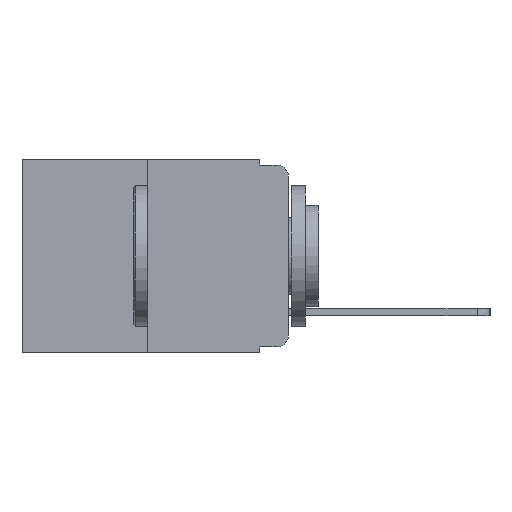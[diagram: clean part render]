
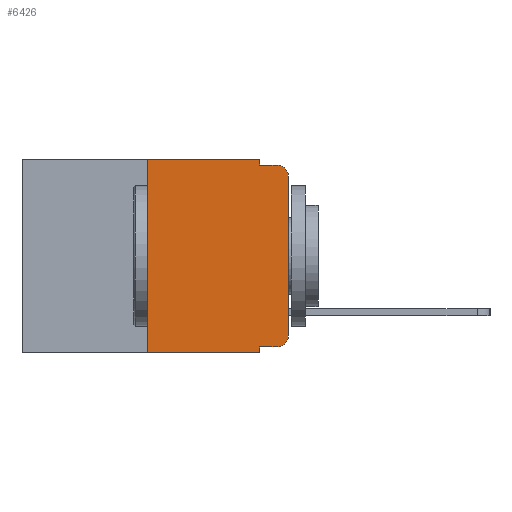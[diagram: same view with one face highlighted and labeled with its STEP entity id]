
A CAD part, left-side view. The second image highlights one B-rep face of the part: STEP entity #6426.
In plain terms, the highlighted planar face has unit normal (-1, 0, 0).
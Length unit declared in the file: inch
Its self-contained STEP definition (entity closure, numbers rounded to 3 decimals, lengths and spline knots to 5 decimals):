
#98 = EDGE_LOOP ( 'NONE', ( #11228, #19823, #4964, #5455, #9560, #14132, #4216, #12463, #16988, #5717 ) ) ;
#233 = CARTESIAN_POINT ( 'NONE',  ( 0., 0.02, -0.01 ) ) ;
#795 = VERTEX_POINT ( 'NONE', #17831 ) ;
#928 = EDGE_CURVE ( 'NONE', #9464, #13873, #5778, .T. ) ;
#1078 = DIRECTION ( 'NONE',  ( 1., 0., 0. ) ) ;
#1104 = VECTOR ( 'NONE', #4983, 39.37008 ) ;
#1154 = VECTOR ( 'NONE', #8101, 39.37008 ) ;
#1570 = LINE ( 'NONE', #16933, #2056 ) ;
#1580 = LINE ( 'NONE', #3253, #1104 ) ;
#1630 = LINE ( 'NONE', #18786, #1154 ) ;
#1838 = DIRECTION ( 'NONE',  ( 0., -1., 0. ) ) ;
#1951 = EDGE_CURVE ( 'NONE', #13873, #5137, #1580, .T. ) ;
#2056 = VECTOR ( 'NONE', #16936, 39.37008 ) ;
#2544 = PLANE ( 'NONE',  #11538 ) ;
#2596 = VECTOR ( 'NONE', #17527, 39.37008 ) ;
#2626 = DIRECTION ( 'NONE',  ( -1., 0., 0. ) ) ;
#2846 = LINE ( 'NONE', #19289, #18240 ) ;
#2942 = DIRECTION ( 'NONE',  ( 0., -1., 0. ) ) ;
#2963 = EDGE_CURVE ( 'NONE', #15920, #5137, #13215, .T. ) ;
#3253 = CARTESIAN_POINT ( 'NONE',  ( 0., 0.051, -0.01 ) ) ;
#3705 = AXIS2_PLACEMENT_3D ( 'NONE', #11559, #11863, #11842 ) ;
#3991 = EDGE_CURVE ( 'NONE', #795, #15920, #1570, .T. ) ;
#4153 = CARTESIAN_POINT ( 'NONE',  ( 0., 0., -0.03 ) ) ;
#4216 = ORIENTED_EDGE ( 'NONE', *, *, #15617, .T. ) ;
#4964 = ORIENTED_EDGE ( 'NONE', *, *, #1951, .F. ) ;
#4983 = DIRECTION ( 'NONE',  ( 0., -1., 0. ) ) ;
#5137 = VERTEX_POINT ( 'NONE', #233 ) ;
#5455 = ORIENTED_EDGE ( 'NONE', *, *, #928, .F. ) ;
#5717 = ORIENTED_EDGE ( 'NONE', *, *, #8567, .T. ) ;
#5778 = LINE ( 'NONE', #17549, #2596 ) ;
#6110 = CARTESIAN_POINT ( 'NONE',  ( 0., 0.473, 0. ) ) ;
#6426 = ADVANCED_FACE ( 'NONE', ( #11651 ), #2544, .F. ) ;
#7258 = VECTOR ( 'NONE', #1838, 39.37008 ) ;
#7268 = CARTESIAN_POINT ( 'NONE',  ( 0., 0.473, 0. ) ) ;
#7919 = VECTOR ( 'NONE', #17334, 39.37008 ) ;
#8100 = CARTESIAN_POINT ( 'NONE',  ( 0., 0.02, -0.333 ) ) ;
#8101 = DIRECTION ( 'NONE',  ( 0., 0., -1. ) ) ;
#8182 = CARTESIAN_POINT ( 'NONE',  ( 0., 0.051, -0.333 ) ) ;
#8341 = CIRCLE ( 'NONE', #19098, 0.02 ) ;
#8567 = EDGE_CURVE ( 'NONE', #12305, #795, #8341, .T. ) ;
#9285 = CARTESIAN_POINT ( 'NONE',  ( 0., 0.25, -0.343 ) ) ;
#9464 = VERTEX_POINT ( 'NONE', #15642 ) ;
#9560 = ORIENTED_EDGE ( 'NONE', *, *, #17837, .F. ) ;
#11228 = ORIENTED_EDGE ( 'NONE', *, *, #3991, .T. ) ;
#11538 = AXIS2_PLACEMENT_3D ( 'NONE', #7268, #1078, #11873 ) ;
#11559 = CARTESIAN_POINT ( 'NONE',  ( 0., 0.02, -0.03 ) ) ;
#11651 = FACE_OUTER_BOUND ( 'NONE', #98, .T. ) ;
#11842 = DIRECTION ( 'NONE',  ( 0., 0., -1. ) ) ;
#11863 = DIRECTION ( 'NONE',  ( -1., 0., 0. ) ) ;
#11873 = DIRECTION ( 'NONE',  ( 0., 0., -1. ) ) ;
#11885 = CARTESIAN_POINT ( 'NONE',  ( 0., 0.02, -0.313 ) ) ;
#11994 = LINE ( 'NONE', #8182, #7919 ) ;
#12085 = LINE ( 'NONE', #6110, #19699 ) ;
#12163 = VERTEX_POINT ( 'NONE', #9285 ) ;
#12305 = VERTEX_POINT ( 'NONE', #8100 ) ;
#12463 = ORIENTED_EDGE ( 'NONE', *, *, #16765, .F. ) ;
#12640 = CARTESIAN_POINT ( 'NONE',  ( 0., 0.473, -0.343 ) ) ;
#12694 = EDGE_CURVE ( 'NONE', #14301, #12305, #11994, .T. ) ;
#12832 = CARTESIAN_POINT ( 'NONE',  ( 0., 0.051, -0.343 ) ) ;
#13215 = CIRCLE ( 'NONE', #3705, 0.02 ) ;
#13421 = CARTESIAN_POINT ( 'NONE',  ( 0., 0.051, -0.01 ) ) ;
#13442 = DIRECTION ( 'NONE',  ( 0., 0., -1. ) ) ;
#13873 = VERTEX_POINT ( 'NONE', #13421 ) ;
#13960 = LINE ( 'NONE', #12640, #7258 ) ;
#14132 = ORIENTED_EDGE ( 'NONE', *, *, #18810, .F. ) ;
#14301 = VERTEX_POINT ( 'NONE', #17393 ) ;
#15617 = EDGE_CURVE ( 'NONE', #12163, #15693, #13960, .T. ) ;
#15642 = CARTESIAN_POINT ( 'NONE',  ( 0., 0.051, 0. ) ) ;
#15693 = VERTEX_POINT ( 'NONE', #12832 ) ;
#15920 = VERTEX_POINT ( 'NONE', #4153 ) ;
#16765 = EDGE_CURVE ( 'NONE', #14301, #15693, #1630, .T. ) ;
#16933 = CARTESIAN_POINT ( 'NONE',  ( 0., 0., 0. ) ) ;
#16936 = DIRECTION ( 'NONE',  ( 0., 0., 1. ) ) ;
#16988 = ORIENTED_EDGE ( 'NONE', *, *, #12694, .T. ) ;
#17029 = CARTESIAN_POINT ( 'NONE',  ( 0., 0.25, 0. ) ) ;
#17334 = DIRECTION ( 'NONE',  ( 0., -1., 0. ) ) ;
#17393 = CARTESIAN_POINT ( 'NONE',  ( 0., 0.051, -0.333 ) ) ;
#17527 = DIRECTION ( 'NONE',  ( 0., 0., -1. ) ) ;
#17549 = CARTESIAN_POINT ( 'NONE',  ( 0., 0.051, 0. ) ) ;
#17785 = DIRECTION ( 'NONE',  ( 0., 0., 1. ) ) ;
#17831 = CARTESIAN_POINT ( 'NONE',  ( 0., 0., -0.313 ) ) ;
#17837 = EDGE_CURVE ( 'NONE', #19114, #9464, #12085, .T. ) ;
#18240 = VECTOR ( 'NONE', #17785, 39.37008 ) ;
#18786 = CARTESIAN_POINT ( 'NONE',  ( 0., 0.051, 0. ) ) ;
#18810 = EDGE_CURVE ( 'NONE', #12163, #19114, #2846, .T. ) ;
#19098 = AXIS2_PLACEMENT_3D ( 'NONE', #11885, #2626, #13442 ) ;
#19114 = VERTEX_POINT ( 'NONE', #17029 ) ;
#19289 = CARTESIAN_POINT ( 'NONE',  ( 0., 0.25, 0. ) ) ;
#19699 = VECTOR ( 'NONE', #2942, 39.37008 ) ;
#19823 = ORIENTED_EDGE ( 'NONE', *, *, #2963, .T. ) ;
